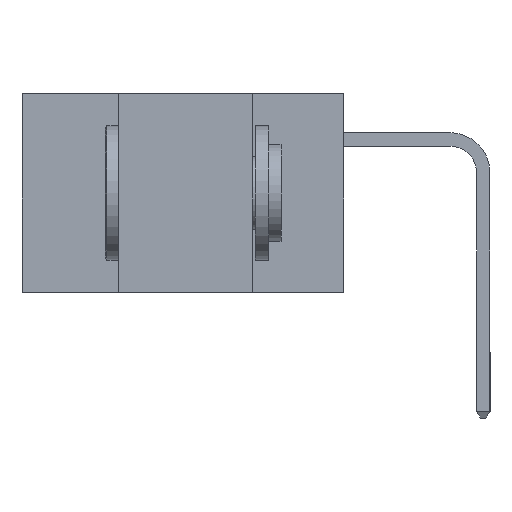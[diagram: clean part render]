
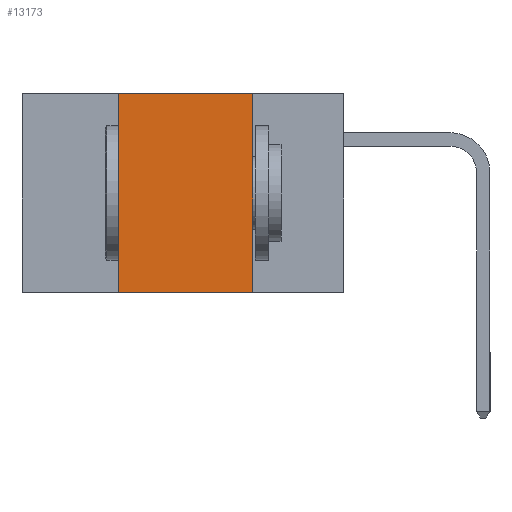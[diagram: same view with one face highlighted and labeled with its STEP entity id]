
A CAD part, left-side view. The second image highlights one B-rep face of the part: STEP entity #13173.
In plain terms, the highlighted planar face has unit normal (-1, 0, 0).
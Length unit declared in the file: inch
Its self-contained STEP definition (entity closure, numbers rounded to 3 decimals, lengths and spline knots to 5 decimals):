
#292 = LINE ( 'NONE', #28278, #5942 ) ;
#481 = CARTESIAN_POINT ( 'NONE',  ( 0., 0.6, 0. ) ) ;
#1400 = CARTESIAN_POINT ( 'NONE',  ( 0., 0.42, 0. ) ) ;
#3405 = DIRECTION ( 'NONE',  ( 1., 0., 0. ) ) ;
#4092 = VERTEX_POINT ( 'NONE', #27924 ) ;
#4168 = AXIS2_PLACEMENT_3D ( 'NONE', #17775, #3405, #20149 ) ;
#4254 = ORIENTED_EDGE ( 'NONE', *, *, #25483, .F. ) ;
#4650 = CARTESIAN_POINT ( 'NONE',  ( 0., 0.42, -0.37 ) ) ;
#5942 = VECTOR ( 'NONE', #9240, 39.37008 ) ;
#7406 = EDGE_CURVE ( 'NONE', #24865, #11374, #292, .T. ) ;
#7909 = DIRECTION ( 'NONE',  ( 0., -1., 0. ) ) ;
#7919 = VECTOR ( 'NONE', #19661, 39.37008 ) ;
#9240 = DIRECTION ( 'NONE',  ( 0., 0., -1. ) ) ;
#10230 = LINE ( 'NONE', #22243, #22928 ) ;
#11200 = CARTESIAN_POINT ( 'NONE',  ( 0., 0.17, 0. ) ) ;
#11374 = VERTEX_POINT ( 'NONE', #13481 ) ;
#12168 = ORIENTED_EDGE ( 'NONE', *, *, #19251, .T. ) ;
#12813 = FACE_OUTER_BOUND ( 'NONE', #26286, .T. ) ;
#13173 = ADVANCED_FACE ( 'NONE', ( #12813 ), #14961, .F. ) ;
#13188 = ORIENTED_EDGE ( 'NONE', *, *, #20551, .F. ) ;
#13481 = CARTESIAN_POINT ( 'NONE',  ( 0., 0.17, -0.37 ) ) ;
#14961 = PLANE ( 'NONE',  #4168 ) ;
#15812 = DIRECTION ( 'NONE',  ( 0., 0., 1. ) ) ;
#17775 = CARTESIAN_POINT ( 'NONE',  ( 0., 0.6, 0. ) ) ;
#19251 = EDGE_CURVE ( 'NONE', #22266, #11374, #10230, .T. ) ;
#19661 = DIRECTION ( 'NONE',  ( 0., -1., 0. ) ) ;
#20149 = DIRECTION ( 'NONE',  ( 0., 0., -1. ) ) ;
#20551 = EDGE_CURVE ( 'NONE', #4092, #24865, #21393, .T. ) ;
#21393 = LINE ( 'NONE', #481, #7919 ) ;
#22243 = CARTESIAN_POINT ( 'NONE',  ( 0., 0.6, -0.37 ) ) ;
#22266 = VERTEX_POINT ( 'NONE', #4650 ) ;
#22928 = VECTOR ( 'NONE', #7909, 39.37008 ) ;
#23105 = LINE ( 'NONE', #1400, #23857 ) ;
#23857 = VECTOR ( 'NONE', #15812, 39.37008 ) ;
#24865 = VERTEX_POINT ( 'NONE', #11200 ) ;
#25483 = EDGE_CURVE ( 'NONE', #22266, #4092, #23105, .T. ) ;
#26286 = EDGE_LOOP ( 'NONE', ( #30581, #13188, #4254, #12168 ) ) ;
#27924 = CARTESIAN_POINT ( 'NONE',  ( 0., 0.42, 0. ) ) ;
#28278 = CARTESIAN_POINT ( 'NONE',  ( 0., 0.17, 0. ) ) ;
#30581 = ORIENTED_EDGE ( 'NONE', *, *, #7406, .F. ) ;
